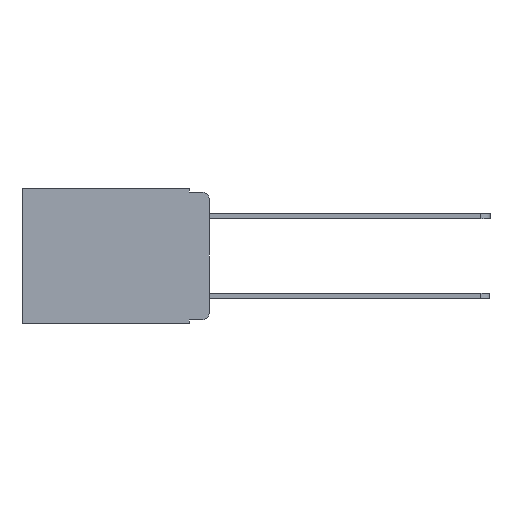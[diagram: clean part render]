
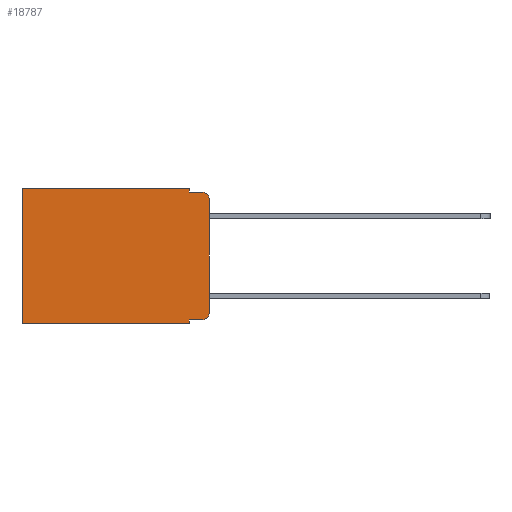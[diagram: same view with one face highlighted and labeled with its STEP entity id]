
A CAD part, left-side view. The second image highlights one B-rep face of the part: STEP entity #18787.
In plain terms, the highlighted planar face has unit normal (-1, 0, 0).
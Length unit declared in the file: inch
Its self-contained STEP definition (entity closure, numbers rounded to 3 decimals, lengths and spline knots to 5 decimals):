
#16 = LINE ( 'NONE', #14627, #4840 ) ;
#402 = EDGE_CURVE ( 'NONE', #23298, #15032, #4076, .T. ) ;
#542 = DIRECTION ( 'NONE',  ( 0., -1., 0. ) ) ;
#623 = ORIENTED_EDGE ( 'NONE', *, *, #19040, .T. ) ;
#635 = VECTOR ( 'NONE', #1058, 39.37008 ) ;
#1058 = DIRECTION ( 'NONE',  ( 0., -1., 0. ) ) ;
#1069 = VERTEX_POINT ( 'NONE', #7129 ) ;
#1332 = DIRECTION ( 'NONE',  ( 1., 0., 0. ) ) ;
#1557 = EDGE_CURVE ( 'NONE', #8608, #1069, #12375, .T. ) ;
#2014 = ORIENTED_EDGE ( 'NONE', *, *, #20931, .F. ) ;
#2954 = EDGE_CURVE ( 'NONE', #15032, #17378, #17342, .T. ) ;
#2975 = ORIENTED_EDGE ( 'NONE', *, *, #10390, .T. ) ;
#3588 = AXIS2_PLACEMENT_3D ( 'NONE', #6175, #19643, #8139 ) ;
#3646 = DIRECTION ( 'NONE',  ( -1., 0., 0. ) ) ;
#3783 = EDGE_CURVE ( 'NONE', #23298, #17738, #10088, .T. ) ;
#4076 = LINE ( 'NONE', #11311, #18924 ) ;
#4633 = ORIENTED_EDGE ( 'NONE', *, *, #16063, .F. ) ;
#4840 = VECTOR ( 'NONE', #16517, 39.37008 ) ;
#4894 = ORIENTED_EDGE ( 'NONE', *, *, #3783, .F. ) ;
#5141 = EDGE_CURVE ( 'NONE', #17738, #11327, #16336, .T. ) ;
#5970 = AXIS2_PLACEMENT_3D ( 'NONE', #15350, #3646, #17236 ) ;
#6022 = CARTESIAN_POINT ( 'NONE',  ( 0.298, 0.051, 0. ) ) ;
#6175 = CARTESIAN_POINT ( 'NONE',  ( 0.298, 0.02, -0.313 ) ) ;
#6468 = ORIENTED_EDGE ( 'NONE', *, *, #2954, .T. ) ;
#7129 = CARTESIAN_POINT ( 'NONE',  ( 0.298, 0.051, -0.343 ) ) ;
#7873 = CARTESIAN_POINT ( 'NONE',  ( 0.298, 0.051, -0.333 ) ) ;
#8139 = DIRECTION ( 'NONE',  ( 0., 0., -1. ) ) ;
#8141 = CIRCLE ( 'NONE', #3588, 0.02 ) ;
#8255 = CARTESIAN_POINT ( 'NONE',  ( 0.298, 0.02, -0.01 ) ) ;
#8292 = CARTESIAN_POINT ( 'NONE',  ( 0.298, 0., -0.03 ) ) ;
#8515 = CARTESIAN_POINT ( 'NONE',  ( 0.298, 0.051, -0.333 ) ) ;
#8608 = VERTEX_POINT ( 'NONE', #7873 ) ;
#9646 = DIRECTION ( 'NONE',  ( 0., 0., -1. ) ) ;
#10088 = LINE ( 'NONE', #17439, #24677 ) ;
#10193 = DIRECTION ( 'NONE',  ( 0., 1., 0. ) ) ;
#10390 = EDGE_CURVE ( 'NONE', #18353, #11327, #17269, .T. ) ;
#11311 = CARTESIAN_POINT ( 'NONE',  ( 0.298, 0., 0. ) ) ;
#11327 = VERTEX_POINT ( 'NONE', #8255 ) ;
#12021 = AXIS2_PLACEMENT_3D ( 'NONE', #24514, #1332, #15109 ) ;
#12245 = ORIENTED_EDGE ( 'NONE', *, *, #1557, .F. ) ;
#12375 = LINE ( 'NONE', #19277, #21823 ) ;
#13450 = ORIENTED_EDGE ( 'NONE', *, *, #402, .T. ) ;
#13548 = LINE ( 'NONE', #23690, #18594 ) ;
#13799 = ORIENTED_EDGE ( 'NONE', *, *, #20286, .T. ) ;
#14292 = DIRECTION ( 'NONE',  ( 0., 0., -1. ) ) ;
#14295 = DIRECTION ( 'NONE',  ( 0., 0., -1. ) ) ;
#14627 = CARTESIAN_POINT ( 'NONE',  ( 0.298, 0., -0.343 ) ) ;
#15032 = VERTEX_POINT ( 'NONE', #16323 ) ;
#15109 = DIRECTION ( 'NONE',  ( 0., 0., -1. ) ) ;
#15350 = CARTESIAN_POINT ( 'NONE',  ( 0.298, 0.02, -0.03 ) ) ;
#16063 = EDGE_CURVE ( 'NONE', #1069, #17378, #16, .T. ) ;
#16269 = CARTESIAN_POINT ( 'NONE',  ( 0.298, 0.051, -0.01 ) ) ;
#16323 = CARTESIAN_POINT ( 'NONE',  ( 0.298, 0.473, 0. ) ) ;
#16336 = LINE ( 'NONE', #20361, #635 ) ;
#16517 = DIRECTION ( 'NONE',  ( 0., 1., 0. ) ) ;
#17014 = CARTESIAN_POINT ( 'NONE',  ( 0.298, 0.473, -0.343 ) ) ;
#17236 = DIRECTION ( 'NONE',  ( 0., 0., -1. ) ) ;
#17269 = CIRCLE ( 'NONE', #5970, 0.02 ) ;
#17342 = LINE ( 'NONE', #22176, #21758 ) ;
#17378 = VERTEX_POINT ( 'NONE', #17014 ) ;
#17439 = CARTESIAN_POINT ( 'NONE',  ( 0.298, 0.051, 0. ) ) ;
#17702 = VECTOR ( 'NONE', #542, 39.37008 ) ;
#17738 = VERTEX_POINT ( 'NONE', #16269 ) ;
#18079 = CARTESIAN_POINT ( 'NONE',  ( 0.298, 0.02, -0.333 ) ) ;
#18225 = CARTESIAN_POINT ( 'NONE',  ( 0.298, 0., -0.313 ) ) ;
#18353 = VERTEX_POINT ( 'NONE', #8292 ) ;
#18594 = VECTOR ( 'NONE', #14295, 39.37008 ) ;
#18787 = ADVANCED_FACE ( 'NONE', ( #19482 ), #20719, .F. ) ;
#18924 = VECTOR ( 'NONE', #10193, 39.37008 ) ;
#19040 = EDGE_CURVE ( 'NONE', #19145, #19730, #8141, .T. ) ;
#19084 = ORIENTED_EDGE ( 'NONE', *, *, #5141, .F. ) ;
#19145 = VERTEX_POINT ( 'NONE', #18079 ) ;
#19277 = CARTESIAN_POINT ( 'NONE',  ( 0.298, 0.051, 0. ) ) ;
#19482 = FACE_OUTER_BOUND ( 'NONE', #22386, .T. ) ;
#19643 = DIRECTION ( 'NONE',  ( -1., 0., 0. ) ) ;
#19730 = VERTEX_POINT ( 'NONE', #18225 ) ;
#20286 = EDGE_CURVE ( 'NONE', #8608, #19145, #22720, .T. ) ;
#20361 = CARTESIAN_POINT ( 'NONE',  ( 0.298, 0.051, -0.01 ) ) ;
#20719 = PLANE ( 'NONE',  #12021 ) ;
#20931 = EDGE_CURVE ( 'NONE', #18353, #19730, #13548, .T. ) ;
#21758 = VECTOR ( 'NONE', #9646, 39.37008 ) ;
#21823 = VECTOR ( 'NONE', #24728, 39.37008 ) ;
#22176 = CARTESIAN_POINT ( 'NONE',  ( 0.298, 0.473, 0. ) ) ;
#22386 = EDGE_LOOP ( 'NONE', ( #2014, #2975, #19084, #4894, #13450, #6468, #4633, #12245, #13799, #623 ) ) ;
#22720 = LINE ( 'NONE', #8515, #17702 ) ;
#23298 = VERTEX_POINT ( 'NONE', #6022 ) ;
#23690 = CARTESIAN_POINT ( 'NONE',  ( 0.298, 0., 0. ) ) ;
#24514 = CARTESIAN_POINT ( 'NONE',  ( 0.298, 0., 0. ) ) ;
#24677 = VECTOR ( 'NONE', #14292, 39.37008 ) ;
#24728 = DIRECTION ( 'NONE',  ( 0., 0., -1. ) ) ;
